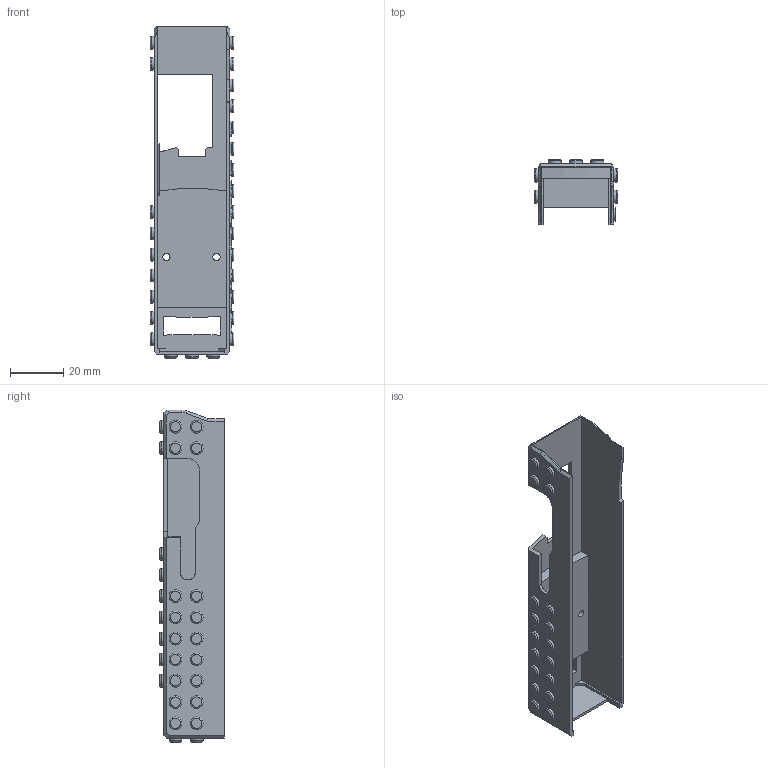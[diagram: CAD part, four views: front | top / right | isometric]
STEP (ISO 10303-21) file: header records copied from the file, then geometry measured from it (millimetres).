
FILE_DESCRIPTION(/* description */ ('Unknown'),/* implementation_level */ '2;1');
FILE_NAME(/* name */ 'MEGAGLOCK SLIDE COVER',/* time_stamp */ '2021-07-15T19:28:26-04:00',/* author */ ('Unknown'),/* organization */ ('Unknown'),/* preprocessor_version */ 'ST-DEVELOPER v16.7',/* originating_system */ 'DEX',/* authorisation */ $);
FILE_SCHEMA (('AUTOMOTIVE_DESIGN {1 0 10303 214 3 1 1}'));
Length unit declared in the file: millimetre
Products named in the file (1): slide cover
Bounding box: 31.54 x 24.27 x 124.73 mm (x, y, z)
Volume: 17109.3 mm3; surface area: 17976.4 mm2
Topology: 2 solids, 2 shells, 448 faces, 1049 edges, 697 vertices
Faces by surface type: plane 246, cylinder 93, torus 79, bspline 24, cone 6
Full cylindrical faces by diameter (mm): 2.705 x2, 4.8 x79
Entity records: 12152 total; most frequent: CARTESIAN_POINT 2907, DIRECTION 1876, ORIENTED_EDGE 1606, EDGE_CURVE 803, EDGE_LOOP 712, FACE_BOUND 712, AXIS2_PLACEMENT_3D 696, VERTEX_POINT 615
